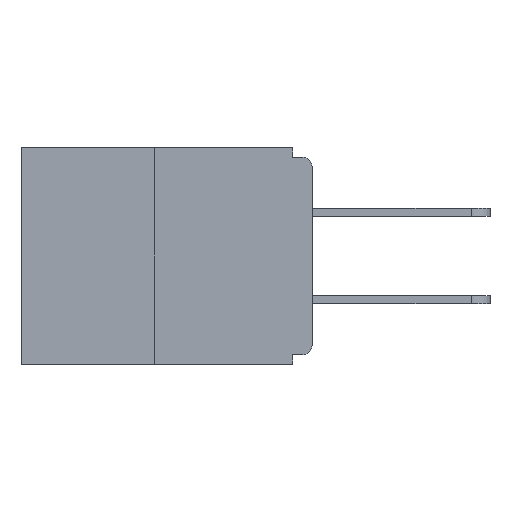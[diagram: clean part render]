
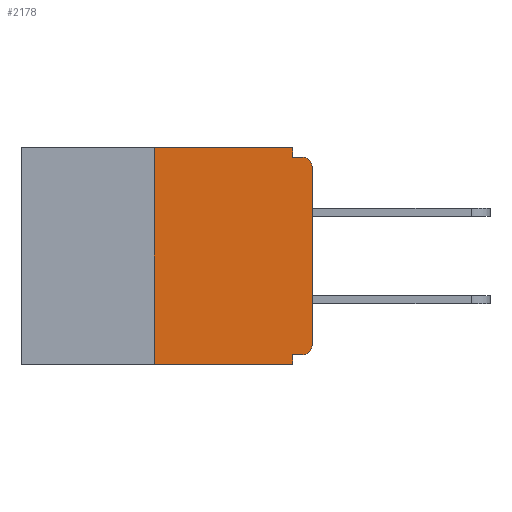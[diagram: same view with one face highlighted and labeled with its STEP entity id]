
A CAD part, left-side view. The second image highlights one B-rep face of the part: STEP entity #2178.
In plain terms, the highlighted planar face has unit normal (-1, 0, 0).
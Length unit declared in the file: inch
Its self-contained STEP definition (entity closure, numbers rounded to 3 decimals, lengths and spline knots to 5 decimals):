
#350 = EDGE_CURVE ( 'NONE', #10124, #25308, #5121, .T. ) ;
#713 = CARTESIAN_POINT ( 'NONE',  ( 0., 0.031, -0.015 ) ) ;
#823 = EDGE_CURVE ( 'NONE', #21123, #25308, #2193, .T. ) ;
#826 = EDGE_CURVE ( 'NONE', #22504, #5259, #18985, .T. ) ;
#946 = VERTEX_POINT ( 'NONE', #9247 ) ;
#2116 = CARTESIAN_POINT ( 'NONE',  ( 0., 0.25, 0. ) ) ;
#2178 = ADVANCED_FACE ( 'NONE', ( #18518 ), #11152, .F. ) ;
#2193 = CIRCLE ( 'NONE', #11258, 0.015 ) ;
#2714 = CARTESIAN_POINT ( 'NONE',  ( 0., 0.46, 0. ) ) ;
#2930 = DIRECTION ( 'NONE',  ( 0., 0., 1. ) ) ;
#3349 = CARTESIAN_POINT ( 'NONE',  ( 0., 0.015, -0.313 ) ) ;
#4173 = AXIS2_PLACEMENT_3D ( 'NONE', #3349, #12354, #12561 ) ;
#4794 = EDGE_CURVE ( 'NONE', #22504, #9290, #11839, .T. ) ;
#5121 = LINE ( 'NONE', #22280, #10269 ) ;
#5259 = VERTEX_POINT ( 'NONE', #25336 ) ;
#7148 = CARTESIAN_POINT ( 'NONE',  ( 0., 0.015, -0.015 ) ) ;
#7624 = EDGE_LOOP ( 'NONE', ( #27886, #30004, #8490, #8162, #23883, #25346, #24158, #13039, #21473, #20034 ) ) ;
#7879 = VECTOR ( 'NONE', #2930, 39.37008 ) ;
#8115 = EDGE_CURVE ( 'NONE', #20057, #25993, #9881, .T. ) ;
#8162 = ORIENTED_EDGE ( 'NONE', *, *, #21850, .F. ) ;
#8490 = ORIENTED_EDGE ( 'NONE', *, *, #826, .T. ) ;
#9014 = DIRECTION ( 'NONE',  ( 1., 0., 0. ) ) ;
#9247 = CARTESIAN_POINT ( 'NONE',  ( 0., 0.031, 0. ) ) ;
#9268 = DIRECTION ( 'NONE',  ( 0., 0., 1. ) ) ;
#9290 = VERTEX_POINT ( 'NONE', #25832 ) ;
#9630 = EDGE_CURVE ( 'NONE', #20057, #27821, #15544, .T. ) ;
#9744 = LINE ( 'NONE', #28508, #18855 ) ;
#9769 = DIRECTION ( 'NONE',  ( 0., -1., 0. ) ) ;
#9881 = CIRCLE ( 'NONE', #4173, 0.015 ) ;
#10124 = VERTEX_POINT ( 'NONE', #713 ) ;
#10200 = CARTESIAN_POINT ( 'NONE',  ( 0., 0.46, -0.343 ) ) ;
#10269 = VECTOR ( 'NONE', #17769, 39.37008 ) ;
#11152 = PLANE ( 'NONE',  #15336 ) ;
#11258 = AXIS2_PLACEMENT_3D ( 'NONE', #14865, #21931, #12643 ) ;
#11839 = LINE ( 'NONE', #2116, #26830 ) ;
#12010 = CARTESIAN_POINT ( 'NONE',  ( 0., 0., -0.313 ) ) ;
#12354 = DIRECTION ( 'NONE',  ( -1., 0., 0. ) ) ;
#12561 = DIRECTION ( 'NONE',  ( 0., 0., -1. ) ) ;
#12643 = DIRECTION ( 'NONE',  ( 0., 0., -1. ) ) ;
#13039 = ORIENTED_EDGE ( 'NONE', *, *, #823, .T. ) ;
#13348 = CARTESIAN_POINT ( 'NONE',  ( 0., 0.031, -0.328 ) ) ;
#13361 = LINE ( 'NONE', #2714, #18818 ) ;
#14752 = CARTESIAN_POINT ( 'NONE',  ( 0., 0., 0. ) ) ;
#14865 = CARTESIAN_POINT ( 'NONE',  ( 0., 0.015, -0.03 ) ) ;
#15336 = AXIS2_PLACEMENT_3D ( 'NONE', #25342, #9014, #20535 ) ;
#15544 = LINE ( 'NONE', #17321, #26933 ) ;
#16315 = DIRECTION ( 'NONE',  ( 0., 0., -1. ) ) ;
#16976 = EDGE_CURVE ( 'NONE', #9290, #946, #13361, .T. ) ;
#17321 = CARTESIAN_POINT ( 'NONE',  ( 0., 0., -0.328 ) ) ;
#17769 = DIRECTION ( 'NONE',  ( 0., -1., 0. ) ) ;
#18518 = FACE_OUTER_BOUND ( 'NONE', #7624, .T. ) ;
#18818 = VECTOR ( 'NONE', #9769, 39.37008 ) ;
#18855 = VECTOR ( 'NONE', #26016, 39.37008 ) ;
#18985 = LINE ( 'NONE', #10200, #21570 ) ;
#19521 = CARTESIAN_POINT ( 'NONE',  ( 0., 0.25, -0.343 ) ) ;
#20034 = ORIENTED_EDGE ( 'NONE', *, *, #25681, .F. ) ;
#20057 = VERTEX_POINT ( 'NONE', #29015 ) ;
#20535 = DIRECTION ( 'NONE',  ( 0., 0., -1. ) ) ;
#21123 = VERTEX_POINT ( 'NONE', #26327 ) ;
#21473 = ORIENTED_EDGE ( 'NONE', *, *, #350, .F. ) ;
#21570 = VECTOR ( 'NONE', #28938, 39.37008 ) ;
#21740 = DIRECTION ( 'NONE',  ( 0., 1., 0. ) ) ;
#21850 = EDGE_CURVE ( 'NONE', #27821, #5259, #9744, .T. ) ;
#21931 = DIRECTION ( 'NONE',  ( -1., 0., 0. ) ) ;
#22044 = EDGE_CURVE ( 'NONE', #25993, #21123, #28785, .T. ) ;
#22280 = CARTESIAN_POINT ( 'NONE',  ( 0., 0., -0.015 ) ) ;
#22504 = VERTEX_POINT ( 'NONE', #19521 ) ;
#23475 = LINE ( 'NONE', #25945, #29712 ) ;
#23883 = ORIENTED_EDGE ( 'NONE', *, *, #9630, .F. ) ;
#24158 = ORIENTED_EDGE ( 'NONE', *, *, #22044, .T. ) ;
#25308 = VERTEX_POINT ( 'NONE', #7148 ) ;
#25336 = CARTESIAN_POINT ( 'NONE',  ( 0., 0.031, -0.343 ) ) ;
#25342 = CARTESIAN_POINT ( 'NONE',  ( 0., 0.46, 0. ) ) ;
#25346 = ORIENTED_EDGE ( 'NONE', *, *, #8115, .T. ) ;
#25681 = EDGE_CURVE ( 'NONE', #946, #10124, #23475, .T. ) ;
#25832 = CARTESIAN_POINT ( 'NONE',  ( 0., 0.25, 0. ) ) ;
#25945 = CARTESIAN_POINT ( 'NONE',  ( 0., 0.031, 0. ) ) ;
#25993 = VERTEX_POINT ( 'NONE', #12010 ) ;
#26016 = DIRECTION ( 'NONE',  ( 0., 0., -1. ) ) ;
#26327 = CARTESIAN_POINT ( 'NONE',  ( 0., 0., -0.03 ) ) ;
#26830 = VECTOR ( 'NONE', #9268, 39.37008 ) ;
#26933 = VECTOR ( 'NONE', #21740, 39.37008 ) ;
#27821 = VERTEX_POINT ( 'NONE', #13348 ) ;
#27886 = ORIENTED_EDGE ( 'NONE', *, *, #16976, .F. ) ;
#28508 = CARTESIAN_POINT ( 'NONE',  ( 0., 0.031, -0.343 ) ) ;
#28785 = LINE ( 'NONE', #14752, #7879 ) ;
#28938 = DIRECTION ( 'NONE',  ( 0., -1., 0. ) ) ;
#29015 = CARTESIAN_POINT ( 'NONE',  ( 0., 0.015, -0.328 ) ) ;
#29712 = VECTOR ( 'NONE', #16315, 39.37008 ) ;
#30004 = ORIENTED_EDGE ( 'NONE', *, *, #4794, .F. ) ;
